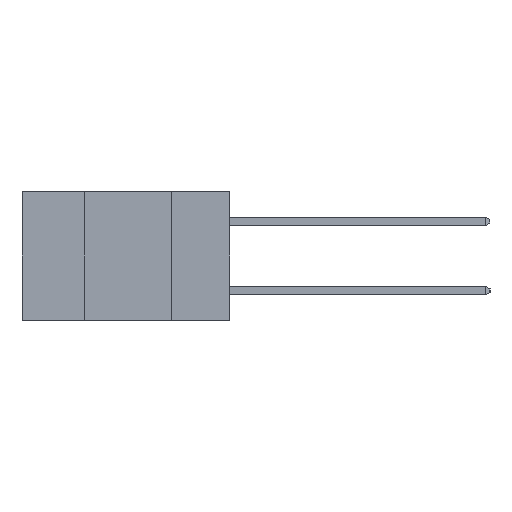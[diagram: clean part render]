
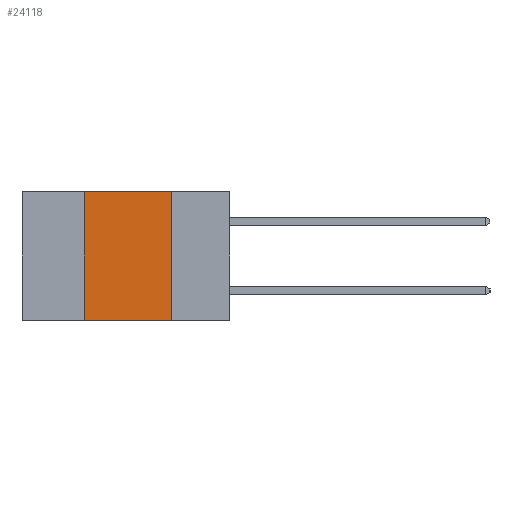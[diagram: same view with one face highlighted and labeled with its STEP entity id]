
A CAD part, left-side view. The second image highlights one B-rep face of the part: STEP entity #24118.
In plain terms, the highlighted planar face has unit normal (-1, 0, 0).
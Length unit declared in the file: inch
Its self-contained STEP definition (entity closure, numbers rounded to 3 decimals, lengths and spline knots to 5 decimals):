
#218 = ORIENTED_EDGE ( 'NONE', *, *, #664, .F. ) ;
#664 = EDGE_CURVE ( 'NONE', #3861, #14753, #4723, .T. ) ;
#1676 = ORIENTED_EDGE ( 'NONE', *, *, #10623, .T. ) ;
#2028 = CARTESIAN_POINT ( 'NONE',  ( 0., 0.17, -0.37 ) ) ;
#2217 = FACE_OUTER_BOUND ( 'NONE', #10268, .T. ) ;
#3321 = VECTOR ( 'NONE', #7012, 39.37008 ) ;
#3861 = VERTEX_POINT ( 'NONE', #24926 ) ;
#4723 = LINE ( 'NONE', #21181, #24998 ) ;
#5155 = EDGE_CURVE ( 'NONE', #14753, #19954, #8859, .T. ) ;
#5998 = PLANE ( 'NONE',  #24664 ) ;
#6144 = CARTESIAN_POINT ( 'NONE',  ( 0., 0.6, -0.37 ) ) ;
#7012 = DIRECTION ( 'NONE',  ( 0., -1., 0. ) ) ;
#7073 = CARTESIAN_POINT ( 'NONE',  ( 0., 0.6, 0. ) ) ;
#8094 = DIRECTION ( 'NONE',  ( 1., 0., 0. ) ) ;
#8859 = LINE ( 'NONE', #7073, #3321 ) ;
#10268 = EDGE_LOOP ( 'NONE', ( #16857, #15914, #218, #1676 ) ) ;
#10623 = EDGE_CURVE ( 'NONE', #3861, #12178, #19916, .T. ) ;
#12178 = VERTEX_POINT ( 'NONE', #2028 ) ;
#13188 = DIRECTION ( 'NONE',  ( 0., 0., -1. ) ) ;
#14165 = CARTESIAN_POINT ( 'NONE',  ( 0., 0.6, 0. ) ) ;
#14753 = VERTEX_POINT ( 'NONE', #15910 ) ;
#15910 = CARTESIAN_POINT ( 'NONE',  ( 0., 0.42, 0. ) ) ;
#15914 = ORIENTED_EDGE ( 'NONE', *, *, #5155, .F. ) ;
#16857 = ORIENTED_EDGE ( 'NONE', *, *, #24474, .F. ) ;
#18672 = VECTOR ( 'NONE', #24350, 39.37008 ) ;
#19256 = CARTESIAN_POINT ( 'NONE',  ( 0., 0.17, -0.37 ) ) ;
#19916 = LINE ( 'NONE', #6144, #18672 ) ;
#19954 = VERTEX_POINT ( 'NONE', #22099 ) ;
#20407 = LINE ( 'NONE', #19256, #25037 ) ;
#21115 = DIRECTION ( 'NONE',  ( 0., 0., 1. ) ) ;
#21181 = CARTESIAN_POINT ( 'NONE',  ( 0., 0.42, -0.37 ) ) ;
#22099 = CARTESIAN_POINT ( 'NONE',  ( 0., 0.17, 0. ) ) ;
#22249 = DIRECTION ( 'NONE',  ( 0., 0., -1. ) ) ;
#24118 = ADVANCED_FACE ( 'NONE', ( #2217 ), #5998, .F. ) ;
#24350 = DIRECTION ( 'NONE',  ( 0., -1., 0. ) ) ;
#24474 = EDGE_CURVE ( 'NONE', #19954, #12178, #20407, .T. ) ;
#24664 = AXIS2_PLACEMENT_3D ( 'NONE', #14165, #8094, #22249 ) ;
#24926 = CARTESIAN_POINT ( 'NONE',  ( 0., 0.42, -0.37 ) ) ;
#24998 = VECTOR ( 'NONE', #21115, 39.37008 ) ;
#25037 = VECTOR ( 'NONE', #13188, 39.37008 ) ;
